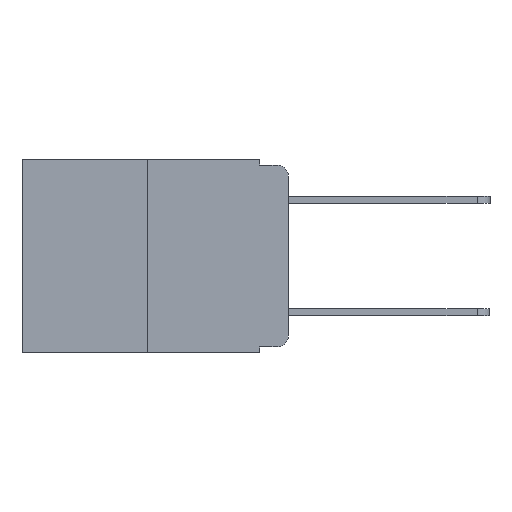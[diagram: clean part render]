
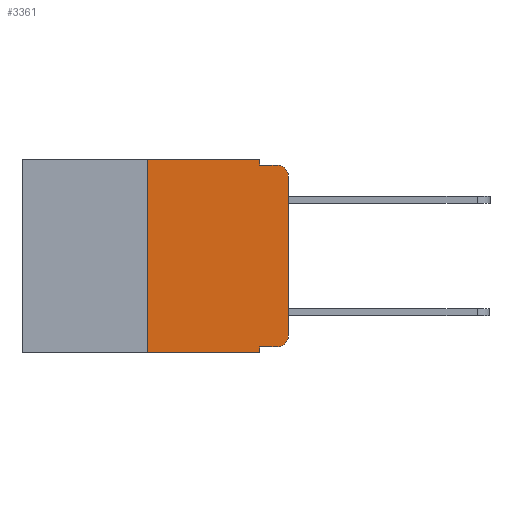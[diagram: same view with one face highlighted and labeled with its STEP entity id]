
A CAD part, left-side view. The second image highlights one B-rep face of the part: STEP entity #3361.
In plain terms, the highlighted planar face has unit normal (-1, 0, 0).
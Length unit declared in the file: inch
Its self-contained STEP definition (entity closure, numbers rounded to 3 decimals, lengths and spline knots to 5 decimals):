
#54 = ORIENTED_EDGE ( 'NONE', *, *, #1453, .F. ) ;
#258 = CARTESIAN_POINT ( 'NONE',  ( 0., 0.02, -0.01 ) ) ;
#349 = CARTESIAN_POINT ( 'NONE',  ( 0., 0., -0.313 ) ) ;
#515 = CIRCLE ( 'NONE', #2269, 0.02 ) ;
#1081 = LINE ( 'NONE', #10751, #3257 ) ;
#1158 = VECTOR ( 'NONE', #4878, 39.37008 ) ;
#1221 = EDGE_CURVE ( 'NONE', #9676, #8392, #6609, .T. ) ;
#1243 = ORIENTED_EDGE ( 'NONE', *, *, #11559, .T. ) ;
#1266 = VERTEX_POINT ( 'NONE', #258 ) ;
#1453 = EDGE_CURVE ( 'NONE', #1801, #3733, #8588, .T. ) ;
#1603 = VECTOR ( 'NONE', #9320, 39.37008 ) ;
#1801 = VERTEX_POINT ( 'NONE', #5234 ) ;
#2021 = CARTESIAN_POINT ( 'NONE',  ( 0., 0.473, 0. ) ) ;
#2165 = ORIENTED_EDGE ( 'NONE', *, *, #11953, .T. ) ;
#2269 = AXIS2_PLACEMENT_3D ( 'NONE', #10603, #5064, #11523 ) ;
#2490 = VECTOR ( 'NONE', #3227, 39.37008 ) ;
#2554 = ORIENTED_EDGE ( 'NONE', *, *, #5130, .T. ) ;
#2794 = CIRCLE ( 'NONE', #11152, 0.02 ) ;
#2863 = VERTEX_POINT ( 'NONE', #7752 ) ;
#2955 = DIRECTION ( 'NONE',  ( 0., 0., -1. ) ) ;
#3166 = VERTEX_POINT ( 'NONE', #5370 ) ;
#3227 = DIRECTION ( 'NONE',  ( 0., -1., 0. ) ) ;
#3257 = VECTOR ( 'NONE', #9872, 39.37008 ) ;
#3282 = CARTESIAN_POINT ( 'NONE',  ( 0., 0.473, 0. ) ) ;
#3361 = ADVANCED_FACE ( 'NONE', ( #4490 ), #5742, .F. ) ;
#3425 = CARTESIAN_POINT ( 'NONE',  ( 0., 0.051, -0.01 ) ) ;
#3446 = ORIENTED_EDGE ( 'NONE', *, *, #6315, .F. ) ;
#3572 = EDGE_CURVE ( 'NONE', #3621, #5903, #7136, .T. ) ;
#3621 = VERTEX_POINT ( 'NONE', #7965 ) ;
#3720 = CARTESIAN_POINT ( 'NONE',  ( 0., 0.25, 0. ) ) ;
#3733 = VERTEX_POINT ( 'NONE', #3425 ) ;
#3844 = EDGE_CURVE ( 'NONE', #3733, #1266, #4483, .T. ) ;
#3985 = VECTOR ( 'NONE', #8850, 39.37008 ) ;
#4128 = CARTESIAN_POINT ( 'NONE',  ( 0., 0.25, 0. ) ) ;
#4483 = LINE ( 'NONE', #8286, #11281 ) ;
#4490 = FACE_OUTER_BOUND ( 'NONE', #4592, .T. ) ;
#4591 = CARTESIAN_POINT ( 'NONE',  ( 0., 0.25, -0.343 ) ) ;
#4592 = EDGE_LOOP ( 'NONE', ( #2554, #1243, #11278, #54, #3446, #11420, #7708, #9412, #2165, #8007 ) ) ;
#4632 = VECTOR ( 'NONE', #10637, 39.37008 ) ;
#4735 = VECTOR ( 'NONE', #6277, 39.37008 ) ;
#4878 = DIRECTION ( 'NONE',  ( 0., 0., -1. ) ) ;
#5064 = DIRECTION ( 'NONE',  ( -1., 0., 0. ) ) ;
#5065 = CARTESIAN_POINT ( 'NONE',  ( 0., 0.051, 0. ) ) ;
#5072 = CARTESIAN_POINT ( 'NONE',  ( 0., 0.051, -0.333 ) ) ;
#5130 = EDGE_CURVE ( 'NONE', #7546, #2863, #11800, .T. ) ;
#5234 = CARTESIAN_POINT ( 'NONE',  ( 0., 0.051, 0. ) ) ;
#5370 = CARTESIAN_POINT ( 'NONE',  ( 0., 0.02, -0.333 ) ) ;
#5391 = CARTESIAN_POINT ( 'NONE',  ( 0., 0.051, 0. ) ) ;
#5457 = DIRECTION ( 'NONE',  ( -1., 0., 0. ) ) ;
#5742 = PLANE ( 'NONE',  #7934 ) ;
#5903 = VERTEX_POINT ( 'NONE', #10989 ) ;
#6277 = DIRECTION ( 'NONE',  ( 0., 0., 1. ) ) ;
#6315 = EDGE_CURVE ( 'NONE', #8392, #1801, #6488, .T. ) ;
#6488 = LINE ( 'NONE', #3282, #3985 ) ;
#6609 = LINE ( 'NONE', #4128, #1603 ) ;
#7136 = LINE ( 'NONE', #5065, #4632 ) ;
#7546 = VERTEX_POINT ( 'NONE', #349 ) ;
#7708 = ORIENTED_EDGE ( 'NONE', *, *, #10056, .T. ) ;
#7752 = CARTESIAN_POINT ( 'NONE',  ( 0., 0., -0.03 ) ) ;
#7934 = AXIS2_PLACEMENT_3D ( 'NONE', #2021, #8530, #2955 ) ;
#7965 = CARTESIAN_POINT ( 'NONE',  ( 0., 0.051, -0.333 ) ) ;
#8007 = ORIENTED_EDGE ( 'NONE', *, *, #8046, .T. ) ;
#8046 = EDGE_CURVE ( 'NONE', #3166, #7546, #515, .T. ) ;
#8286 = CARTESIAN_POINT ( 'NONE',  ( 0., 0.051, -0.01 ) ) ;
#8392 = VERTEX_POINT ( 'NONE', #3720 ) ;
#8530 = DIRECTION ( 'NONE',  ( 1., 0., 0. ) ) ;
#8588 = LINE ( 'NONE', #5391, #1158 ) ;
#8850 = DIRECTION ( 'NONE',  ( 0., -1., 0. ) ) ;
#9192 = DIRECTION ( 'NONE',  ( 0., -1., 0. ) ) ;
#9320 = DIRECTION ( 'NONE',  ( 0., 0., 1. ) ) ;
#9412 = ORIENTED_EDGE ( 'NONE', *, *, #3572, .F. ) ;
#9676 = VERTEX_POINT ( 'NONE', #4591 ) ;
#9872 = DIRECTION ( 'NONE',  ( 0., -1., 0. ) ) ;
#9889 = LINE ( 'NONE', #5072, #2490 ) ;
#10056 = EDGE_CURVE ( 'NONE', #9676, #5903, #1081, .T. ) ;
#10603 = CARTESIAN_POINT ( 'NONE',  ( 0., 0.02, -0.313 ) ) ;
#10637 = DIRECTION ( 'NONE',  ( 0., 0., -1. ) ) ;
#10751 = CARTESIAN_POINT ( 'NONE',  ( 0., 0.473, -0.343 ) ) ;
#10979 = CARTESIAN_POINT ( 'NONE',  ( 0., 0.02, -0.03 ) ) ;
#10989 = CARTESIAN_POINT ( 'NONE',  ( 0., 0.051, -0.343 ) ) ;
#11152 = AXIS2_PLACEMENT_3D ( 'NONE', #10979, #5457, #11902 ) ;
#11278 = ORIENTED_EDGE ( 'NONE', *, *, #3844, .F. ) ;
#11281 = VECTOR ( 'NONE', #9192, 39.37008 ) ;
#11420 = ORIENTED_EDGE ( 'NONE', *, *, #1221, .F. ) ;
#11523 = DIRECTION ( 'NONE',  ( 0., 0., -1. ) ) ;
#11559 = EDGE_CURVE ( 'NONE', #2863, #1266, #2794, .T. ) ;
#11756 = CARTESIAN_POINT ( 'NONE',  ( 0., 0., 0. ) ) ;
#11800 = LINE ( 'NONE', #11756, #4735 ) ;
#11902 = DIRECTION ( 'NONE',  ( 0., 0., -1. ) ) ;
#11953 = EDGE_CURVE ( 'NONE', #3621, #3166, #9889, .T. ) ;
